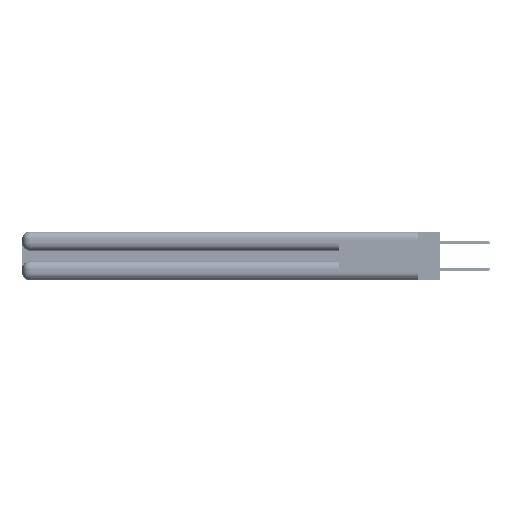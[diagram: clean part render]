
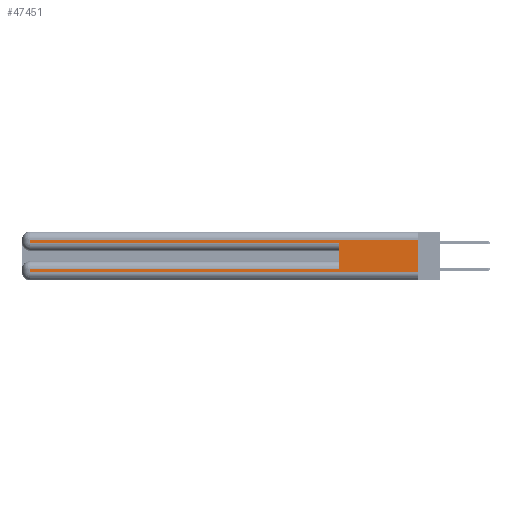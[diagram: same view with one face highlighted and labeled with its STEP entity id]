
A CAD part, left-side view. The second image highlights one B-rep face of the part: STEP entity #47451.
In plain terms, the highlighted planar face has unit normal (-1, 0, 0).
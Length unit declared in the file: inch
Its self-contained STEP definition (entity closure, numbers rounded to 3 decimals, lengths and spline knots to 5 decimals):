
#42 = CARTESIAN_POINT ( 'NONE',  ( 0., 2.94, 0.285 ) ) ;
#74 = DIRECTION ( 'NONE',  ( 0., 0., -1. ) ) ;
#498 = VERTEX_POINT ( 'NONE', #21186 ) ;
#1172 = DIRECTION ( 'NONE',  ( 0., -1., 0. ) ) ;
#3264 = ORIENTED_EDGE ( 'NONE', *, *, #11510, .F. ) ;
#5648 = CARTESIAN_POINT ( 'NONE',  ( 0., 2.94, 0.085 ) ) ;
#6214 = DIRECTION ( 'NONE',  ( 1., 0., 0. ) ) ;
#6274 = VERTEX_POINT ( 'NONE', #42 ) ;
#6295 = CARTESIAN_POINT ( 'NONE',  ( 0., 0., 0.085 ) ) ;
#6395 = PLANE ( 'NONE',  #9220 ) ;
#7356 = EDGE_CURVE ( 'NONE', #6274, #19444, #12763, .T. ) ;
#7549 = LINE ( 'NONE', #28075, #47002 ) ;
#9220 = AXIS2_PLACEMENT_3D ( 'NONE', #18102, #6214, #35180 ) ;
#11510 = EDGE_CURVE ( 'NONE', #14885, #15429, #13033, .T. ) ;
#11695 = ORIENTED_EDGE ( 'NONE', *, *, #13817, .T. ) ;
#12763 = LINE ( 'NONE', #20399, #28020 ) ;
#13033 = LINE ( 'NONE', #32468, #44851 ) ;
#13345 = CARTESIAN_POINT ( 'NONE',  ( 0., 0., 0.06 ) ) ;
#13817 = EDGE_CURVE ( 'NONE', #50995, #15429, #40599, .T. ) ;
#14885 = VERTEX_POINT ( 'NONE', #20541 ) ;
#15062 = EDGE_CURVE ( 'NONE', #20863, #19444, #48114, .T. ) ;
#15429 = VERTEX_POINT ( 'NONE', #39894 ) ;
#17677 = ORIENTED_EDGE ( 'NONE', *, *, #39825, .T. ) ;
#18053 = CARTESIAN_POINT ( 'NONE',  ( 0., 2.94, 0.37 ) ) ;
#18055 = ORIENTED_EDGE ( 'NONE', *, *, #15062, .F. ) ;
#18102 = CARTESIAN_POINT ( 'NONE',  ( 0., 0., 0.37 ) ) ;
#18581 = DIRECTION ( 'NONE',  ( 0., 0., -1. ) ) ;
#19444 = VERTEX_POINT ( 'NONE', #23099 ) ;
#19894 = CARTESIAN_POINT ( 'NONE',  ( 0., 0.6, 0.085 ) ) ;
#20399 = CARTESIAN_POINT ( 'NONE',  ( 0., 0., 0.285 ) ) ;
#20541 = CARTESIAN_POINT ( 'NONE',  ( 0., 0., 0.31 ) ) ;
#20764 = DIRECTION ( 'NONE',  ( 0., -1., 0. ) ) ;
#20863 = VERTEX_POINT ( 'NONE', #19894 ) ;
#21186 = CARTESIAN_POINT ( 'NONE',  ( 0., 2.94, 0.31 ) ) ;
#23099 = CARTESIAN_POINT ( 'NONE',  ( 0., 0.6, 0.285 ) ) ;
#24662 = DIRECTION ( 'NONE',  ( 0., 0., -1. ) ) ;
#26221 = VERTEX_POINT ( 'NONE', #5648 ) ;
#26599 = CARTESIAN_POINT ( 'NONE',  ( 0., 0., 0.31 ) ) ;
#27371 = EDGE_CURVE ( 'NONE', #498, #6274, #46467, .T. ) ;
#28020 = VECTOR ( 'NONE', #20764, 39.37008 ) ;
#28075 = CARTESIAN_POINT ( 'NONE',  ( 0., 2.94, 0.37 ) ) ;
#28532 = FACE_OUTER_BOUND ( 'NONE', #40971, .T. ) ;
#30145 = EDGE_CURVE ( 'NONE', #14885, #498, #52325, .T. ) ;
#32468 = CARTESIAN_POINT ( 'NONE',  ( 0., 0., 0.37 ) ) ;
#32595 = EDGE_CURVE ( 'NONE', #20863, #26221, #47580, .T. ) ;
#33695 = CARTESIAN_POINT ( 'NONE',  ( 0., 0.6, 0.145 ) ) ;
#34428 = DIRECTION ( 'NONE',  ( 0., 1., 0. ) ) ;
#34925 = ORIENTED_EDGE ( 'NONE', *, *, #30145, .T. ) ;
#35084 = CARTESIAN_POINT ( 'NONE',  ( 0., 2.94, 0.06 ) ) ;
#35180 = DIRECTION ( 'NONE',  ( 0., 0., -1. ) ) ;
#35508 = ORIENTED_EDGE ( 'NONE', *, *, #27371, .T. ) ;
#36735 = ORIENTED_EDGE ( 'NONE', *, *, #32595, .T. ) ;
#36902 = VECTOR ( 'NONE', #18581, 39.37008 ) ;
#37314 = VECTOR ( 'NONE', #41718, 39.37008 ) ;
#38493 = DIRECTION ( 'NONE',  ( 0., 1., 0. ) ) ;
#39825 = EDGE_CURVE ( 'NONE', #26221, #50995, #7549, .T. ) ;
#39894 = CARTESIAN_POINT ( 'NONE',  ( 0., 0., 0.06 ) ) ;
#40599 = LINE ( 'NONE', #13345, #51430 ) ;
#40971 = EDGE_LOOP ( 'NONE', ( #3264, #34925, #35508, #41463, #18055, #36735, #17677, #11695 ) ) ;
#41463 = ORIENTED_EDGE ( 'NONE', *, *, #7356, .T. ) ;
#41718 = DIRECTION ( 'NONE',  ( 0., 0., 1. ) ) ;
#44851 = VECTOR ( 'NONE', #24662, 39.37008 ) ;
#45956 = VECTOR ( 'NONE', #34428, 39.37008 ) ;
#46467 = LINE ( 'NONE', #18053, #36902 ) ;
#47002 = VECTOR ( 'NONE', #74, 39.37008 ) ;
#47451 = ADVANCED_FACE ( 'NONE', ( #28532 ), #6395, .F. ) ;
#47580 = LINE ( 'NONE', #6295, #48845 ) ;
#48114 = LINE ( 'NONE', #33695, #37314 ) ;
#48845 = VECTOR ( 'NONE', #38493, 39.37008 ) ;
#50995 = VERTEX_POINT ( 'NONE', #35084 ) ;
#51430 = VECTOR ( 'NONE', #1172, 39.37008 ) ;
#52325 = LINE ( 'NONE', #26599, #45956 ) ;
